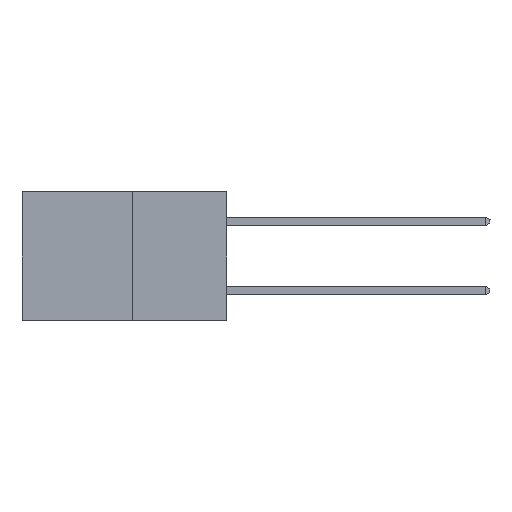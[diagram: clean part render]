
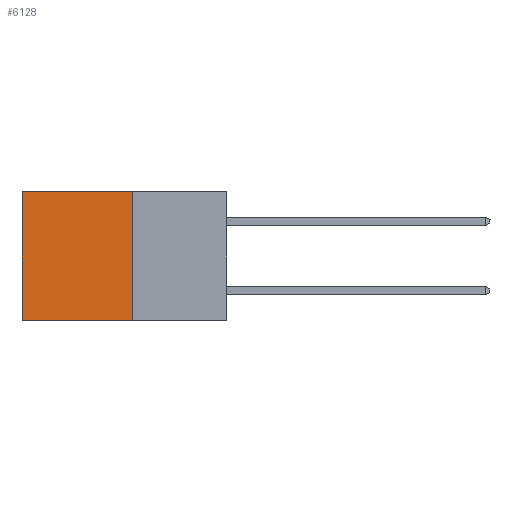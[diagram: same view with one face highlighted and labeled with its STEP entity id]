
A CAD part, left-side view. The second image highlights one B-rep face of the part: STEP entity #6128.
In plain terms, the highlighted planar face has unit normal (-1, 0, 0).
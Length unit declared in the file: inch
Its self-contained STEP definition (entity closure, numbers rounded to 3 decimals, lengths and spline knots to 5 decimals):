
#426 = DIRECTION ( 'NONE',  ( 0., 1., 0. ) ) ;
#473 = CARTESIAN_POINT ( 'NONE',  ( 0.277, 0.27, -0.37 ) ) ;
#3547 = EDGE_LOOP ( 'NONE', ( #8073, #5896, #8572, #8369 ) ) ;
#3906 = VECTOR ( 'NONE', #10145, 39.37008 ) ;
#3925 = AXIS2_PLACEMENT_3D ( 'NONE', #15207, #14950, #14896 ) ;
#4093 = EDGE_CURVE ( 'NONE', #14208, #13616, #13815, .T. ) ;
#5896 = ORIENTED_EDGE ( 'NONE', *, *, #10074, .F. ) ;
#6128 = ADVANCED_FACE ( 'NONE', ( #8391 ), #15002, .F. ) ;
#6317 = EDGE_CURVE ( 'NONE', #10615, #11562, #12285, .T. ) ;
#7166 = VECTOR ( 'NONE', #11434, 39.37008 ) ;
#7912 = CARTESIAN_POINT ( 'NONE',  ( 0.277, 0.59, 0. ) ) ;
#7933 = CARTESIAN_POINT ( 'NONE',  ( 0.277, 0.59, -0.37 ) ) ;
#8073 = ORIENTED_EDGE ( 'NONE', *, *, #4093, .T. ) ;
#8237 = EDGE_CURVE ( 'NONE', #10615, #14208, #11320, .T. ) ;
#8369 = ORIENTED_EDGE ( 'NONE', *, *, #8237, .T. ) ;
#8391 = FACE_OUTER_BOUND ( 'NONE', #3547, .T. ) ;
#8572 = ORIENTED_EDGE ( 'NONE', *, *, #6317, .F. ) ;
#8865 = VECTOR ( 'NONE', #426, 39.37008 ) ;
#9323 = CARTESIAN_POINT ( 'NONE',  ( 0.277, 0.59, -0.37 ) ) ;
#10074 = EDGE_CURVE ( 'NONE', #11562, #13616, #12525, .T. ) ;
#10145 = DIRECTION ( 'NONE',  ( 0., 0., -1. ) ) ;
#10615 = VERTEX_POINT ( 'NONE', #11081 ) ;
#10934 = VECTOR ( 'NONE', #12595, 39.37008 ) ;
#11081 = CARTESIAN_POINT ( 'NONE',  ( 0.277, 0.27, 0. ) ) ;
#11320 = LINE ( 'NONE', #12670, #10934 ) ;
#11434 = DIRECTION ( 'NONE',  ( 0., 0., -1. ) ) ;
#11562 = VERTEX_POINT ( 'NONE', #12626 ) ;
#11601 = CARTESIAN_POINT ( 'NONE',  ( 0.277, 0.27, -0.37 ) ) ;
#12285 = LINE ( 'NONE', #11601, #7166 ) ;
#12525 = LINE ( 'NONE', #473, #8865 ) ;
#12595 = DIRECTION ( 'NONE',  ( 0., 1., 0. ) ) ;
#12626 = CARTESIAN_POINT ( 'NONE',  ( 0.277, 0.27, -0.37 ) ) ;
#12670 = CARTESIAN_POINT ( 'NONE',  ( 0.277, 0.27, 0. ) ) ;
#13616 = VERTEX_POINT ( 'NONE', #7933 ) ;
#13815 = LINE ( 'NONE', #9323, #3906 ) ;
#14208 = VERTEX_POINT ( 'NONE', #7912 ) ;
#14896 = DIRECTION ( 'NONE',  ( 0., 0., -1. ) ) ;
#14950 = DIRECTION ( 'NONE',  ( 1., 0., 0. ) ) ;
#15002 = PLANE ( 'NONE',  #3925 ) ;
#15207 = CARTESIAN_POINT ( 'NONE',  ( 0.277, 0.27, -0.37 ) ) ;
